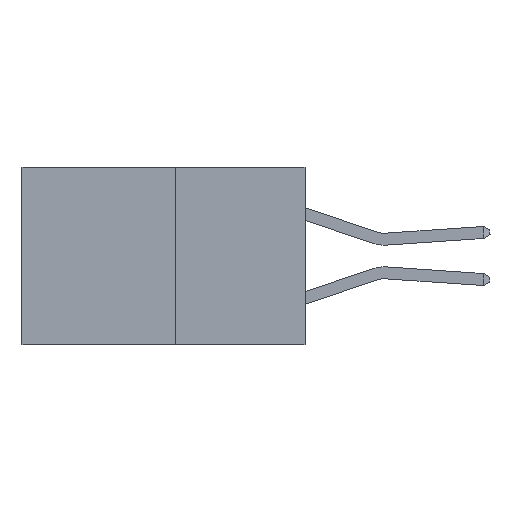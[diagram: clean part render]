
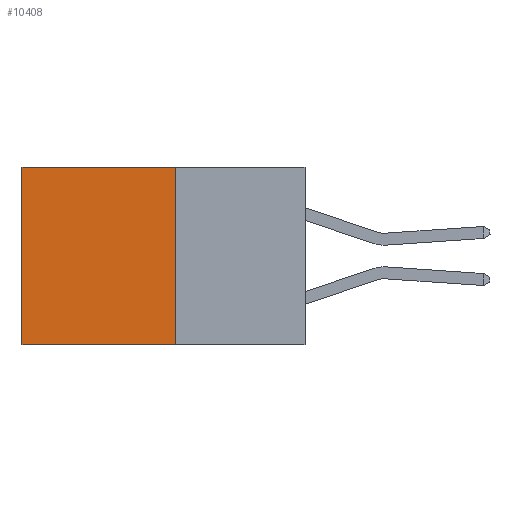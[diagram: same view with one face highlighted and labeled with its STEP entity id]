
A CAD part, left-side view. The second image highlights one B-rep face of the part: STEP entity #10408.
In plain terms, the highlighted planar face has unit normal (-1, 0, 0).
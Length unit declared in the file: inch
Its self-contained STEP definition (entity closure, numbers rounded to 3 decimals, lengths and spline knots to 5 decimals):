
#1055 = DIRECTION ( 'NONE',  ( 1., 0., 0. ) ) ;
#1158 = CARTESIAN_POINT ( 'NONE',  ( 0.277, 0.27, -0.37 ) ) ;
#1169 = AXIS2_PLACEMENT_3D ( 'NONE', #16067, #1055, #9918 ) ;
#1233 = VERTEX_POINT ( 'NONE', #12758 ) ;
#1365 = EDGE_LOOP ( 'NONE', ( #10716, #13644, #9435, #7438 ) ) ;
#2413 = CARTESIAN_POINT ( 'NONE',  ( 0.277, 0.27, -0.37 ) ) ;
#2415 = VECTOR ( 'NONE', #12454, 39.37008 ) ;
#2509 = VECTOR ( 'NONE', #15442, 39.37008 ) ;
#2767 = EDGE_CURVE ( 'NONE', #4250, #14340, #14983, .T. ) ;
#2775 = CARTESIAN_POINT ( 'NONE',  ( 0.277, 0.27, -0.37 ) ) ;
#3195 = EDGE_CURVE ( 'NONE', #1233, #14165, #9168, .T. ) ;
#4022 = FACE_OUTER_BOUND ( 'NONE', #1365, .T. ) ;
#4250 = VERTEX_POINT ( 'NONE', #7702 ) ;
#5749 = DIRECTION ( 'NONE',  ( 0., 0., -1. ) ) ;
#5903 = LINE ( 'NONE', #2413, #2509 ) ;
#6123 = EDGE_CURVE ( 'NONE', #14340, #14165, #5903, .T. ) ;
#6238 = DIRECTION ( 'NONE',  ( 0., 1., 0. ) ) ;
#7438 = ORIENTED_EDGE ( 'NONE', *, *, #13449, .T. ) ;
#7702 = CARTESIAN_POINT ( 'NONE',  ( 0.277, 0.27, 0. ) ) ;
#8401 = VECTOR ( 'NONE', #5749, 39.37008 ) ;
#9168 = LINE ( 'NONE', #10438, #2415 ) ;
#9435 = ORIENTED_EDGE ( 'NONE', *, *, #2767, .F. ) ;
#9918 = DIRECTION ( 'NONE',  ( 0., 0., -1. ) ) ;
#10408 = ADVANCED_FACE ( 'NONE', ( #4022 ), #14826, .F. ) ;
#10438 = CARTESIAN_POINT ( 'NONE',  ( 0.277, 0.59, -0.37 ) ) ;
#10716 = ORIENTED_EDGE ( 'NONE', *, *, #3195, .T. ) ;
#11236 = LINE ( 'NONE', #16199, #14898 ) ;
#12454 = DIRECTION ( 'NONE',  ( 0., 0., -1. ) ) ;
#12758 = CARTESIAN_POINT ( 'NONE',  ( 0.277, 0.59, 0. ) ) ;
#13449 = EDGE_CURVE ( 'NONE', #4250, #1233, #11236, .T. ) ;
#13644 = ORIENTED_EDGE ( 'NONE', *, *, #6123, .F. ) ;
#14165 = VERTEX_POINT ( 'NONE', #16181 ) ;
#14340 = VERTEX_POINT ( 'NONE', #2775 ) ;
#14826 = PLANE ( 'NONE',  #1169 ) ;
#14898 = VECTOR ( 'NONE', #6238, 39.37008 ) ;
#14983 = LINE ( 'NONE', #1158, #8401 ) ;
#15442 = DIRECTION ( 'NONE',  ( 0., 1., 0. ) ) ;
#16067 = CARTESIAN_POINT ( 'NONE',  ( 0.277, 0.27, -0.37 ) ) ;
#16181 = CARTESIAN_POINT ( 'NONE',  ( 0.277, 0.59, -0.37 ) ) ;
#16199 = CARTESIAN_POINT ( 'NONE',  ( 0.277, 0.27, 0. ) ) ;
